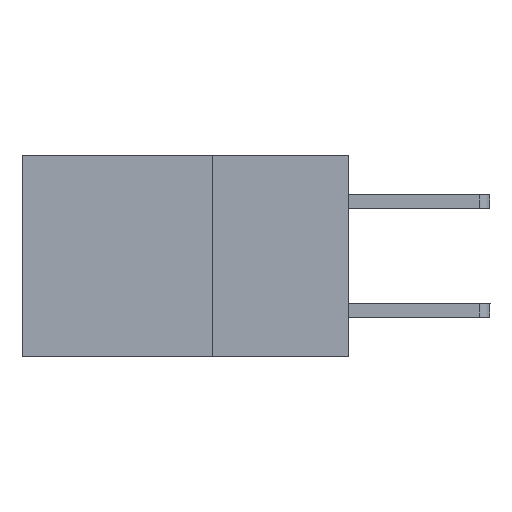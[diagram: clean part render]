
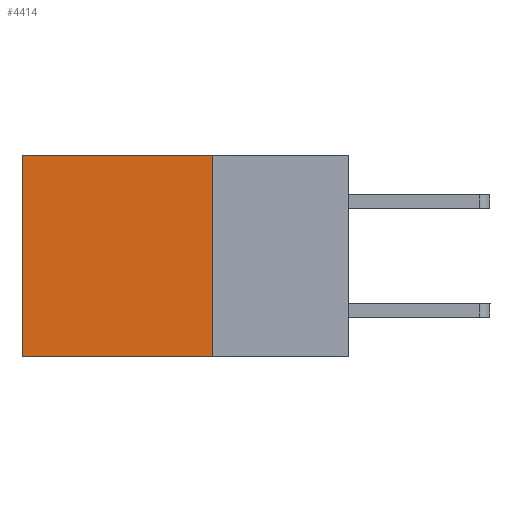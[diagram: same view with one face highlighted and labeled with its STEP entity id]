
A CAD part, left-side view. The second image highlights one B-rep face of the part: STEP entity #4414.
In plain terms, the highlighted planar face has unit normal (-1, 0, 0).
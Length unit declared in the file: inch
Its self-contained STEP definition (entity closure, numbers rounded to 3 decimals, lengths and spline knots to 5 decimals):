
#742 = PLANE ( 'NONE',  #8082 ) ;
#894 = FACE_OUTER_BOUND ( 'NONE', #7775, .T. ) ;
#1143 = VERTEX_POINT ( 'NONE', #10267 ) ;
#1380 = LINE ( 'NONE', #10477, #7505 ) ;
#1445 = CARTESIAN_POINT ( 'NONE',  ( 0.2615, 0.25, -0.37 ) ) ;
#1605 = CARTESIAN_POINT ( 'NONE',  ( 0.2615, 0.25, -0.37 ) ) ;
#1776 = CARTESIAN_POINT ( 'NONE',  ( 0.2615, 0.6, -0.37 ) ) ;
#1811 = EDGE_CURVE ( 'NONE', #1143, #9714, #2610, .T. ) ;
#2441 = DIRECTION ( 'NONE',  ( 0., 0., -1. ) ) ;
#2610 = LINE ( 'NONE', #6975, #8923 ) ;
#3028 = CARTESIAN_POINT ( 'NONE',  ( 0.2615, 0.6, -0.37 ) ) ;
#3374 = EDGE_CURVE ( 'NONE', #4053, #8688, #4548, .T. ) ;
#4053 = VERTEX_POINT ( 'NONE', #4440 ) ;
#4143 = DIRECTION ( 'NONE',  ( 0., 1., 0. ) ) ;
#4414 = ADVANCED_FACE ( 'NONE', ( #894 ), #742, .F. ) ;
#4440 = CARTESIAN_POINT ( 'NONE',  ( 0.2615, 0.6, 0. ) ) ;
#4452 = EDGE_CURVE ( 'NONE', #9714, #8688, #9928, .T. ) ;
#4548 = LINE ( 'NONE', #1776, #6229 ) ;
#4748 = DIRECTION ( 'NONE',  ( 0., 1., 0. ) ) ;
#5383 = ORIENTED_EDGE ( 'NONE', *, *, #4452, .F. ) ;
#6053 = ORIENTED_EDGE ( 'NONE', *, *, #3374, .T. ) ;
#6229 = VECTOR ( 'NONE', #10212, 39.37008 ) ;
#6230 = EDGE_CURVE ( 'NONE', #1143, #4053, #1380, .T. ) ;
#6975 = CARTESIAN_POINT ( 'NONE',  ( 0.2615, 0.25, -0.37 ) ) ;
#6986 = ORIENTED_EDGE ( 'NONE', *, *, #6230, .T. ) ;
#7421 = DIRECTION ( 'NONE',  ( 1., 0., 0. ) ) ;
#7505 = VECTOR ( 'NONE', #4748, 39.37008 ) ;
#7775 = EDGE_LOOP ( 'NONE', ( #6053, #5383, #9493, #6986 ) ) ;
#7911 = DIRECTION ( 'NONE',  ( 0., 0., -1. ) ) ;
#8082 = AXIS2_PLACEMENT_3D ( 'NONE', #1605, #7421, #2441 ) ;
#8688 = VERTEX_POINT ( 'NONE', #3028 ) ;
#8923 = VECTOR ( 'NONE', #7911, 39.37008 ) ;
#9430 = VECTOR ( 'NONE', #4143, 39.37008 ) ;
#9493 = ORIENTED_EDGE ( 'NONE', *, *, #1811, .F. ) ;
#9714 = VERTEX_POINT ( 'NONE', #1445 ) ;
#9839 = CARTESIAN_POINT ( 'NONE',  ( 0.2615, 0.25, -0.37 ) ) ;
#9928 = LINE ( 'NONE', #9839, #9430 ) ;
#10212 = DIRECTION ( 'NONE',  ( 0., 0., -1. ) ) ;
#10267 = CARTESIAN_POINT ( 'NONE',  ( 0.2615, 0.25, 0. ) ) ;
#10477 = CARTESIAN_POINT ( 'NONE',  ( 0.2615, 0.25, 0. ) ) ;
